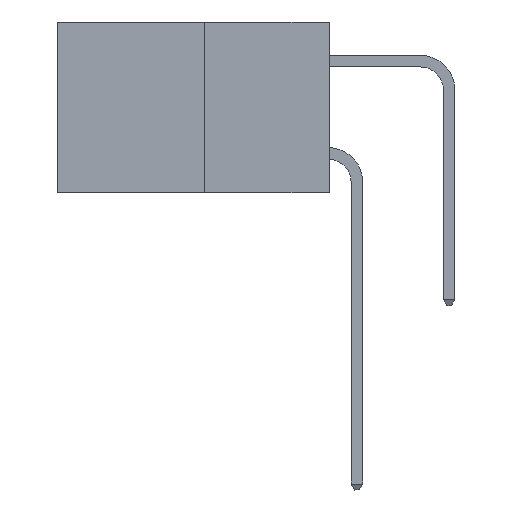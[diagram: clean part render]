
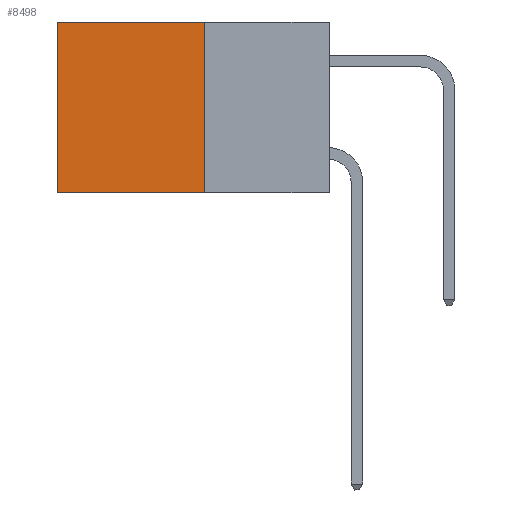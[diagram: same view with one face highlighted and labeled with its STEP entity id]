
A CAD part, left-side view. The second image highlights one B-rep face of the part: STEP entity #8498.
In plain terms, the highlighted planar face has unit normal (-1, 0, 0).
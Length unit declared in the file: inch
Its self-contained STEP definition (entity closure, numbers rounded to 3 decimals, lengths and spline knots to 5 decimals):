
#1478 = CARTESIAN_POINT ( 'NONE',  ( 0.277, 0.59, -0.37 ) ) ;
#1620 = ORIENTED_EDGE ( 'NONE', *, *, #18695, .T. ) ;
#2018 = CARTESIAN_POINT ( 'NONE',  ( 0.277, 0.59, 0. ) ) ;
#2079 = ORIENTED_EDGE ( 'NONE', *, *, #12251, .F. ) ;
#2402 = ORIENTED_EDGE ( 'NONE', *, *, #7670, .F. ) ;
#2818 = ORIENTED_EDGE ( 'NONE', *, *, #17138, .T. ) ;
#4921 = VECTOR ( 'NONE', #25979, 39.37008 ) ;
#7645 = VECTOR ( 'NONE', #29242, 39.37008 ) ;
#7670 = EDGE_CURVE ( 'NONE', #8488, #13229, #9204, .T. ) ;
#8488 = VERTEX_POINT ( 'NONE', #11050 ) ;
#8498 = ADVANCED_FACE ( 'NONE', ( #14845 ), #10760, .F. ) ;
#9204 = LINE ( 'NONE', #25691, #4921 ) ;
#10691 = DIRECTION ( 'NONE',  ( 0., 0., -1. ) ) ;
#10696 = DIRECTION ( 'NONE',  ( 1., 0., 0. ) ) ;
#10760 = PLANE ( 'NONE',  #20737 ) ;
#11050 = CARTESIAN_POINT ( 'NONE',  ( 0.277, 0.27, 0. ) ) ;
#11257 = CARTESIAN_POINT ( 'NONE',  ( 0.277, 0.27, -0.37 ) ) ;
#12251 = EDGE_CURVE ( 'NONE', #13229, #26376, #31147, .T. ) ;
#13229 = VERTEX_POINT ( 'NONE', #31295 ) ;
#14845 = FACE_OUTER_BOUND ( 'NONE', #30546, .T. ) ;
#14942 = CARTESIAN_POINT ( 'NONE',  ( 0.277, 0.27, 0. ) ) ;
#17138 = EDGE_CURVE ( 'NONE', #8488, #24415, #19697, .T. ) ;
#18695 = EDGE_CURVE ( 'NONE', #24415, #26376, #22971, .T. ) ;
#19697 = LINE ( 'NONE', #14942, #7645 ) ;
#19717 = CARTESIAN_POINT ( 'NONE',  ( 0.277, 0.59, -0.37 ) ) ;
#19818 = DIRECTION ( 'NONE',  ( 0., 0., -1. ) ) ;
#20737 = AXIS2_PLACEMENT_3D ( 'NONE', #11257, #10696, #10691 ) ;
#22911 = CARTESIAN_POINT ( 'NONE',  ( 0.277, 0.27, -0.37 ) ) ;
#22971 = LINE ( 'NONE', #19717, #28621 ) ;
#24113 = VECTOR ( 'NONE', #30130, 39.37008 ) ;
#24415 = VERTEX_POINT ( 'NONE', #2018 ) ;
#25691 = CARTESIAN_POINT ( 'NONE',  ( 0.277, 0.27, -0.37 ) ) ;
#25979 = DIRECTION ( 'NONE',  ( 0., 0., -1. ) ) ;
#26376 = VERTEX_POINT ( 'NONE', #1478 ) ;
#28621 = VECTOR ( 'NONE', #19818, 39.37008 ) ;
#29242 = DIRECTION ( 'NONE',  ( 0., 1., 0. ) ) ;
#30130 = DIRECTION ( 'NONE',  ( 0., 1., 0. ) ) ;
#30546 = EDGE_LOOP ( 'NONE', ( #1620, #2079, #2402, #2818 ) ) ;
#31147 = LINE ( 'NONE', #22911, #24113 ) ;
#31295 = CARTESIAN_POINT ( 'NONE',  ( 0.277, 0.27, -0.37 ) ) ;
